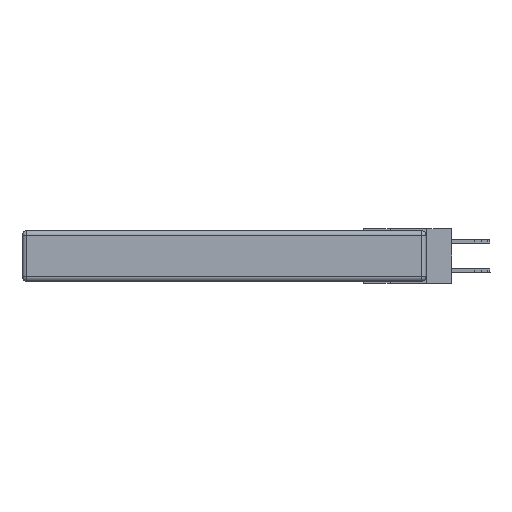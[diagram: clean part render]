
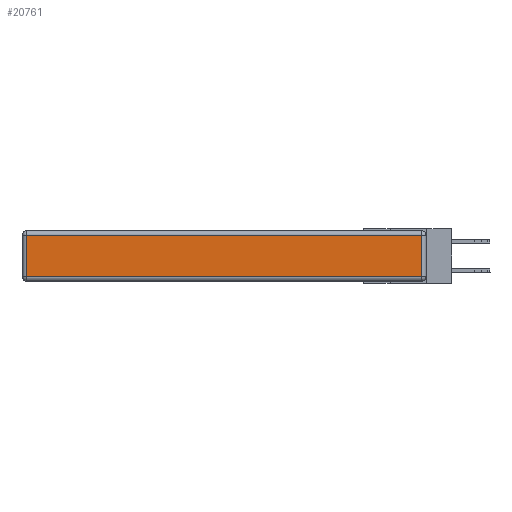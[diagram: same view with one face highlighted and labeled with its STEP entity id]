
A CAD part, left-side view. The second image highlights one B-rep face of the part: STEP entity #20761.
In plain terms, the highlighted planar face has unit normal (-1, 0, 0).
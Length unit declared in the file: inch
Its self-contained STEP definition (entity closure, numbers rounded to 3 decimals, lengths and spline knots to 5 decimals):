
#166 = FACE_OUTER_BOUND ( 'NONE', #10843, .T. ) ;
#338 = CARTESIAN_POINT ( 'NONE',  ( 0., 0.03, -0.313 ) ) ;
#1055 = LINE ( 'NONE', #15779, #8649 ) ;
#2459 = CARTESIAN_POINT ( 'NONE',  ( 0., 2.72, -0.03 ) ) ;
#2682 = EDGE_CURVE ( 'NONE', #19523, #14400, #1055, .T. ) ;
#5003 = VECTOR ( 'NONE', #9180, 39.37008 ) ;
#5293 = EDGE_CURVE ( 'NONE', #14400, #13802, #18061, .T. ) ;
#5441 = ORIENTED_EDGE ( 'NONE', *, *, #22459, .T. ) ;
#6752 = VERTEX_POINT ( 'NONE', #8589 ) ;
#8375 = LINE ( 'NONE', #11163, #22491 ) ;
#8589 = CARTESIAN_POINT ( 'NONE',  ( 0., 2.72, -0.313 ) ) ;
#8649 = VECTOR ( 'NONE', #20792, 39.37008 ) ;
#9180 = DIRECTION ( 'NONE',  ( 0., 1., 0. ) ) ;
#9879 = VECTOR ( 'NONE', #12534, 39.37008 ) ;
#10843 = EDGE_LOOP ( 'NONE', ( #5441, #11038, #16443, #16036 ) ) ;
#11038 = ORIENTED_EDGE ( 'NONE', *, *, #2682, .T. ) ;
#11163 = CARTESIAN_POINT ( 'NONE',  ( 0., 2.72, -0.343 ) ) ;
#12027 = DIRECTION ( 'NONE',  ( 0., 0., 1. ) ) ;
#12237 = CARTESIAN_POINT ( 'NONE',  ( 0., 0., -0.313 ) ) ;
#12534 = DIRECTION ( 'NONE',  ( 0., -1., 0. ) ) ;
#12543 = EDGE_CURVE ( 'NONE', #13802, #6752, #8375, .T. ) ;
#12596 = LINE ( 'NONE', #12237, #9879 ) ;
#12747 = DIRECTION ( 'NONE',  ( 0., 0., -1. ) ) ;
#13481 = AXIS2_PLACEMENT_3D ( 'NONE', #22478, #15445, #12027 ) ;
#13802 = VERTEX_POINT ( 'NONE', #2459 ) ;
#14400 = VERTEX_POINT ( 'NONE', #15821 ) ;
#15445 = DIRECTION ( 'NONE',  ( -1., 0., 0. ) ) ;
#15779 = CARTESIAN_POINT ( 'NONE',  ( 0., 0.03, -0.343 ) ) ;
#15821 = CARTESIAN_POINT ( 'NONE',  ( 0., 0.03, -0.03 ) ) ;
#16036 = ORIENTED_EDGE ( 'NONE', *, *, #12543, .T. ) ;
#16443 = ORIENTED_EDGE ( 'NONE', *, *, #5293, .T. ) ;
#17784 = CARTESIAN_POINT ( 'NONE',  ( 0., 2.75, -0.03 ) ) ;
#18061 = LINE ( 'NONE', #17784, #5003 ) ;
#19523 = VERTEX_POINT ( 'NONE', #338 ) ;
#20761 = ADVANCED_FACE ( 'NONE', ( #166 ), #22398, .T. ) ;
#20792 = DIRECTION ( 'NONE',  ( 0., 0., 1. ) ) ;
#22398 = PLANE ( 'NONE',  #13481 ) ;
#22459 = EDGE_CURVE ( 'NONE', #6752, #19523, #12596, .T. ) ;
#22478 = CARTESIAN_POINT ( 'NONE',  ( 0., 0., -0.343 ) ) ;
#22491 = VECTOR ( 'NONE', #12747, 39.37008 ) ;
